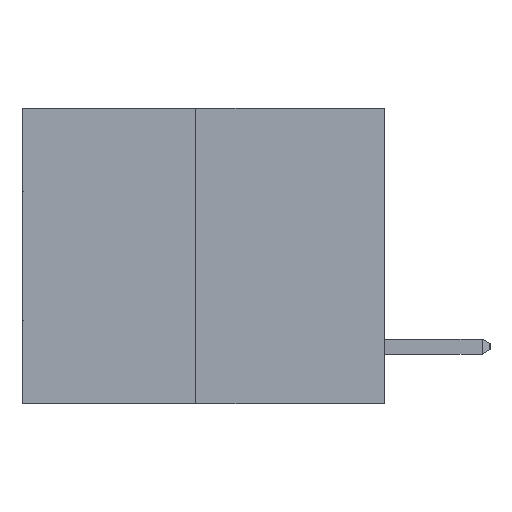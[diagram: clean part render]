
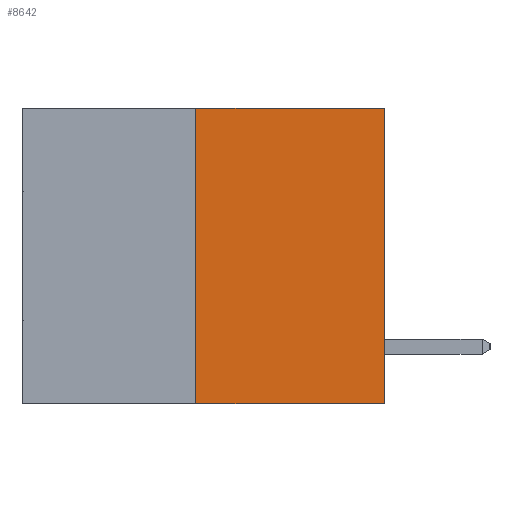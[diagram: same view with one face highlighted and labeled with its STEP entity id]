
A CAD part, left-side view. The second image highlights one B-rep face of the part: STEP entity #8642.
In plain terms, the highlighted planar face has unit normal (-1, 0, 0).
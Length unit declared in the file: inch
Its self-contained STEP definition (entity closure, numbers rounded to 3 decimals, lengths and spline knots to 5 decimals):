
#2172 = VECTOR ( 'NONE', #23282, 39.37008 ) ;
#2562 = AXIS2_PLACEMENT_3D ( 'NONE', #16456, #23663, #3241 ) ;
#3241 = DIRECTION ( 'NONE',  ( 0., 0., -1. ) ) ;
#3540 = EDGE_LOOP ( 'NONE', ( #17921, #26748, #20709, #12149 ) ) ;
#4317 = CARTESIAN_POINT ( 'NONE',  ( 0., 0., 0. ) ) ;
#5046 = VERTEX_POINT ( 'NONE', #8287 ) ;
#6183 = DIRECTION ( 'NONE',  ( 0., 0., 1. ) ) ;
#7991 = EDGE_CURVE ( 'NONE', #19088, #26517, #16241, .T. ) ;
#8287 = CARTESIAN_POINT ( 'NONE',  ( 0., 0.312, -0.49 ) ) ;
#8293 = CARTESIAN_POINT ( 'NONE',  ( 0., 0.312, 0. ) ) ;
#8642 = ADVANCED_FACE ( 'NONE', ( #12132 ), #10991, .F. ) ;
#10991 = PLANE ( 'NONE',  #2562 ) ;
#11798 = VECTOR ( 'NONE', #16645, 39.37008 ) ;
#11908 = CARTESIAN_POINT ( 'NONE',  ( 0., 0.6, 0. ) ) ;
#12132 = FACE_OUTER_BOUND ( 'NONE', #3540, .T. ) ;
#12149 = ORIENTED_EDGE ( 'NONE', *, *, #7991, .F. ) ;
#14866 = DIRECTION ( 'NONE',  ( 0., 0., 1. ) ) ;
#15798 = EDGE_CURVE ( 'NONE', #5046, #19088, #21502, .T. ) ;
#16215 = VECTOR ( 'NONE', #6183, 39.37008 ) ;
#16241 = LINE ( 'NONE', #11908, #11798 ) ;
#16456 = CARTESIAN_POINT ( 'NONE',  ( 0., 0.6, 0. ) ) ;
#16645 = DIRECTION ( 'NONE',  ( 0., -1., 0. ) ) ;
#17921 = ORIENTED_EDGE ( 'NONE', *, *, #15798, .F. ) ;
#18944 = VECTOR ( 'NONE', #14866, 39.37008 ) ;
#19088 = VERTEX_POINT ( 'NONE', #8293 ) ;
#19412 = CARTESIAN_POINT ( 'NONE',  ( 0., 0., -0.49 ) ) ;
#19457 = CARTESIAN_POINT ( 'NONE',  ( 0., 0.312, -0.49 ) ) ;
#20709 = ORIENTED_EDGE ( 'NONE', *, *, #25535, .T. ) ;
#20828 = LINE ( 'NONE', #20832, #2172 ) ;
#20832 = CARTESIAN_POINT ( 'NONE',  ( 0., 0.6, -0.49 ) ) ;
#21502 = LINE ( 'NONE', #19457, #18944 ) ;
#22743 = CARTESIAN_POINT ( 'NONE',  ( 0., 0., 0. ) ) ;
#23282 = DIRECTION ( 'NONE',  ( 0., -1., 0. ) ) ;
#23663 = DIRECTION ( 'NONE',  ( 1., 0., 0. ) ) ;
#25535 = EDGE_CURVE ( 'NONE', #27293, #26517, #25692, .T. ) ;
#25692 = LINE ( 'NONE', #4317, #16215 ) ;
#26517 = VERTEX_POINT ( 'NONE', #22743 ) ;
#26748 = ORIENTED_EDGE ( 'NONE', *, *, #27754, .T. ) ;
#27293 = VERTEX_POINT ( 'NONE', #19412 ) ;
#27754 = EDGE_CURVE ( 'NONE', #5046, #27293, #20828, .T. ) ;
